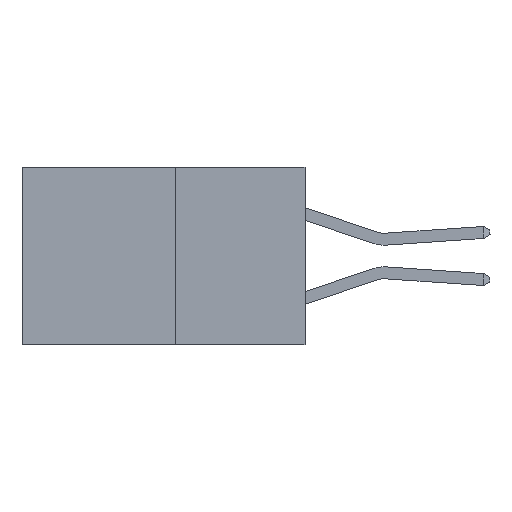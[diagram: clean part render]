
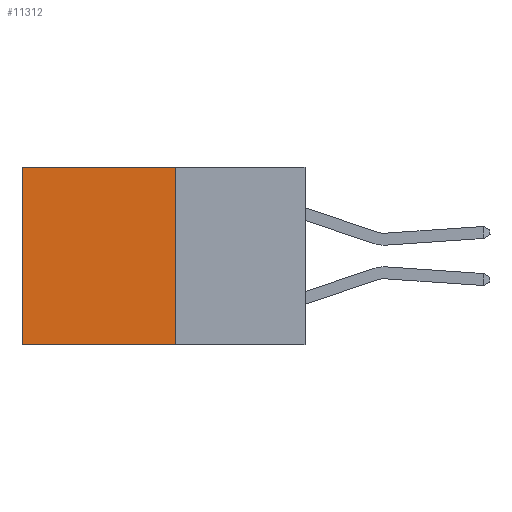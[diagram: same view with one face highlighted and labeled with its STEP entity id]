
A CAD part, left-side view. The second image highlights one B-rep face of the part: STEP entity #11312.
In plain terms, the highlighted planar face has unit normal (-1, 0, 0).
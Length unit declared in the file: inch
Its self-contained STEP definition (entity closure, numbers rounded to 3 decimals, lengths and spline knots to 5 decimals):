
#140 = LINE ( 'NONE', #4788, #6733 ) ;
#147 = CARTESIAN_POINT ( 'NONE',  ( 0.277, 0.59, 0. ) ) ;
#195 = VERTEX_POINT ( 'NONE', #147 ) ;
#522 = CARTESIAN_POINT ( 'NONE',  ( 0.277, 0.59, -0.37 ) ) ;
#1304 = CARTESIAN_POINT ( 'NONE',  ( 0.277, 0.27, -0.37 ) ) ;
#1348 = LINE ( 'NONE', #2234, #15644 ) ;
#1673 = CARTESIAN_POINT ( 'NONE',  ( 0.277, 0.59, -0.37 ) ) ;
#2234 = CARTESIAN_POINT ( 'NONE',  ( 0.277, 0.27, -0.37 ) ) ;
#2740 = DIRECTION ( 'NONE',  ( 0., 0., -1. ) ) ;
#3380 = ORIENTED_EDGE ( 'NONE', *, *, #6782, .F. ) ;
#3672 = EDGE_CURVE ( 'NONE', #6145, #195, #15971, .T. ) ;
#4033 = VERTEX_POINT ( 'NONE', #15479 ) ;
#4098 = ORIENTED_EDGE ( 'NONE', *, *, #14412, .F. ) ;
#4788 = CARTESIAN_POINT ( 'NONE',  ( 0.277, 0.27, -0.37 ) ) ;
#4808 = FACE_OUTER_BOUND ( 'NONE', #12704, .T. ) ;
#6145 = VERTEX_POINT ( 'NONE', #8287 ) ;
#6733 = VECTOR ( 'NONE', #7495, 39.37008 ) ;
#6782 = EDGE_CURVE ( 'NONE', #6145, #4033, #140, .T. ) ;
#6962 = DIRECTION ( 'NONE',  ( 0., 1., 0. ) ) ;
#7409 = VECTOR ( 'NONE', #11400, 39.37008 ) ;
#7495 = DIRECTION ( 'NONE',  ( 0., 0., -1. ) ) ;
#7687 = CARTESIAN_POINT ( 'NONE',  ( 0.277, 0.27, 0. ) ) ;
#8256 = PLANE ( 'NONE',  #10826 ) ;
#8287 = CARTESIAN_POINT ( 'NONE',  ( 0.277, 0.27, 0. ) ) ;
#8552 = ORIENTED_EDGE ( 'NONE', *, *, #17455, .T. ) ;
#10542 = DIRECTION ( 'NONE',  ( 0., 1., 0. ) ) ;
#10826 = AXIS2_PLACEMENT_3D ( 'NONE', #1304, #11033, #2740 ) ;
#11033 = DIRECTION ( 'NONE',  ( 1., 0., 0. ) ) ;
#11060 = LINE ( 'NONE', #1673, #7409 ) ;
#11312 = ADVANCED_FACE ( 'NONE', ( #4808 ), #8256, .F. ) ;
#11400 = DIRECTION ( 'NONE',  ( 0., 0., -1. ) ) ;
#12319 = VECTOR ( 'NONE', #6962, 39.37008 ) ;
#12704 = EDGE_LOOP ( 'NONE', ( #8552, #4098, #3380, #15706 ) ) ;
#14412 = EDGE_CURVE ( 'NONE', #4033, #16934, #1348, .T. ) ;
#15479 = CARTESIAN_POINT ( 'NONE',  ( 0.277, 0.27, -0.37 ) ) ;
#15644 = VECTOR ( 'NONE', #10542, 39.37008 ) ;
#15706 = ORIENTED_EDGE ( 'NONE', *, *, #3672, .T. ) ;
#15971 = LINE ( 'NONE', #7687, #12319 ) ;
#16934 = VERTEX_POINT ( 'NONE', #522 ) ;
#17455 = EDGE_CURVE ( 'NONE', #195, #16934, #11060, .T. ) ;
